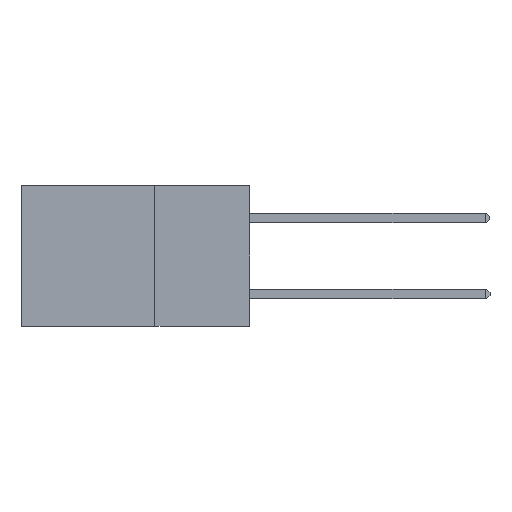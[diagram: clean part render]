
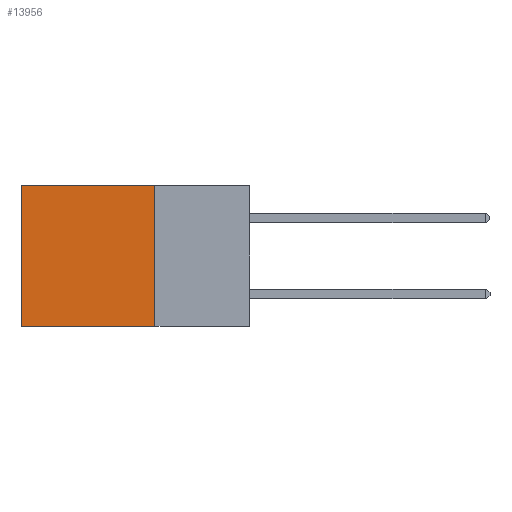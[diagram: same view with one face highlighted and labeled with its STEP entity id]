
A CAD part, left-side view. The second image highlights one B-rep face of the part: STEP entity #13956.
In plain terms, the highlighted planar face has unit normal (-1, 0, 0).
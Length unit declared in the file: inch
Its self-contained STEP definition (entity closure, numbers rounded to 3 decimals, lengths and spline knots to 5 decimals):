
#580 = VECTOR ( 'NONE', #14057, 39.37008 ) ;
#1508 = CARTESIAN_POINT ( 'NONE',  ( 0.2875, 0.25, 0. ) ) ;
#1991 = CARTESIAN_POINT ( 'NONE',  ( 0.2875, 0.6, -0.37 ) ) ;
#2162 = CARTESIAN_POINT ( 'NONE',  ( 0.2875, 0.25, -0.37 ) ) ;
#2268 = ORIENTED_EDGE ( 'NONE', *, *, #4174, .F. ) ;
#2570 = EDGE_LOOP ( 'NONE', ( #7232, #2268, #20350, #5006 ) ) ;
#2788 = PLANE ( 'NONE',  #6256 ) ;
#3079 = CARTESIAN_POINT ( 'NONE',  ( 0.2875, 0.6, 0. ) ) ;
#4174 = EDGE_CURVE ( 'NONE', #21142, #15517, #17068, .T. ) ;
#5006 = ORIENTED_EDGE ( 'NONE', *, *, #6642, .T. ) ;
#6256 = AXIS2_PLACEMENT_3D ( 'NONE', #7910, #19610, #9612 ) ;
#6642 = EDGE_CURVE ( 'NONE', #6828, #9586, #9582, .T. ) ;
#6828 = VERTEX_POINT ( 'NONE', #17861 ) ;
#7232 = ORIENTED_EDGE ( 'NONE', *, *, #17272, .T. ) ;
#7313 = LINE ( 'NONE', #3079, #11820 ) ;
#7472 = LINE ( 'NONE', #1508, #11980 ) ;
#7910 = CARTESIAN_POINT ( 'NONE',  ( 0.2875, 0.25, 0. ) ) ;
#8910 = DIRECTION ( 'NONE',  ( 0., 1., 0. ) ) ;
#9582 = LINE ( 'NONE', #20700, #580 ) ;
#9586 = VERTEX_POINT ( 'NONE', #9900 ) ;
#9612 = DIRECTION ( 'NONE',  ( 0., 0., -1. ) ) ;
#9900 = CARTESIAN_POINT ( 'NONE',  ( 0.2875, 0.6, 0. ) ) ;
#9944 = DIRECTION ( 'NONE',  ( 0., 0., -1. ) ) ;
#10129 = CARTESIAN_POINT ( 'NONE',  ( 0.2875, 0.25, -0.37 ) ) ;
#10287 = EDGE_CURVE ( 'NONE', #6828, #21142, #7472, .T. ) ;
#11820 = VECTOR ( 'NONE', #13204, 39.37008 ) ;
#11980 = VECTOR ( 'NONE', #9944, 39.37008 ) ;
#13204 = DIRECTION ( 'NONE',  ( 0., 0., -1. ) ) ;
#13956 = ADVANCED_FACE ( 'NONE', ( #20158 ), #2788, .F. ) ;
#14057 = DIRECTION ( 'NONE',  ( 0., 1., 0. ) ) ;
#15517 = VERTEX_POINT ( 'NONE', #1991 ) ;
#16079 = VECTOR ( 'NONE', #8910, 39.37008 ) ;
#17068 = LINE ( 'NONE', #2162, #16079 ) ;
#17272 = EDGE_CURVE ( 'NONE', #9586, #15517, #7313, .T. ) ;
#17861 = CARTESIAN_POINT ( 'NONE',  ( 0.2875, 0.25, 0. ) ) ;
#19610 = DIRECTION ( 'NONE',  ( 1., 0., 0. ) ) ;
#20158 = FACE_OUTER_BOUND ( 'NONE', #2570, .T. ) ;
#20350 = ORIENTED_EDGE ( 'NONE', *, *, #10287, .F. ) ;
#20700 = CARTESIAN_POINT ( 'NONE',  ( 0.2875, 0.25, 0. ) ) ;
#21142 = VERTEX_POINT ( 'NONE', #10129 ) ;
